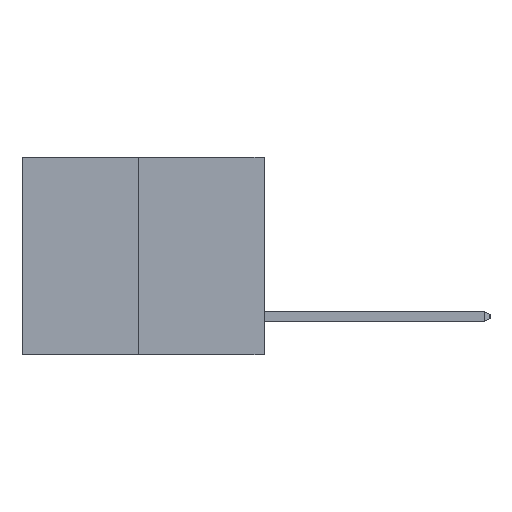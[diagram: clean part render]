
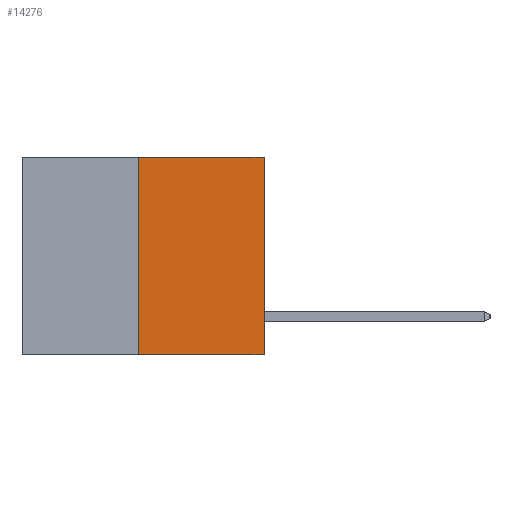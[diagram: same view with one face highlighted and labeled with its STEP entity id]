
A CAD part, left-side view. The second image highlights one B-rep face of the part: STEP entity #14276.
In plain terms, the highlighted planar face has unit normal (-1, 0, 0).
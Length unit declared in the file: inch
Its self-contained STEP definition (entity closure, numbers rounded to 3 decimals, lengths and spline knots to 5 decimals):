
#96 = ORIENTED_EDGE ( 'NONE', *, *, #14423, .F. ) ;
#719 = LINE ( 'NONE', #15150, #18676 ) ;
#1601 = EDGE_CURVE ( 'NONE', #19548, #9227, #719, .T. ) ;
#2883 = LINE ( 'NONE', #22093, #15667 ) ;
#3592 = DIRECTION ( 'NONE',  ( 0., -1., 0. ) ) ;
#3836 = AXIS2_PLACEMENT_3D ( 'NONE', #12516, #15598, #21388 ) ;
#4018 = CARTESIAN_POINT ( 'NONE',  ( 0., 0.312, 0. ) ) ;
#4059 = EDGE_LOOP ( 'NONE', ( #96, #14963, #13814, #21442 ) ) ;
#5556 = PLANE ( 'NONE',  #3836 ) ;
#5925 = VECTOR ( 'NONE', #3592, 39.37008 ) ;
#6572 = EDGE_CURVE ( 'NONE', #9227, #20650, #2883, .T. ) ;
#7530 = FACE_OUTER_BOUND ( 'NONE', #4059, .T. ) ;
#8862 = DIRECTION ( 'NONE',  ( 0., 0., 1. ) ) ;
#9227 = VERTEX_POINT ( 'NONE', #14667 ) ;
#9747 = DIRECTION ( 'NONE',  ( 0., 0., 1. ) ) ;
#10704 = VERTEX_POINT ( 'NONE', #4018 ) ;
#11401 = DIRECTION ( 'NONE',  ( 0., -1., 0. ) ) ;
#12516 = CARTESIAN_POINT ( 'NONE',  ( 0., 0.6, 0. ) ) ;
#13814 = ORIENTED_EDGE ( 'NONE', *, *, #6572, .T. ) ;
#13989 = CARTESIAN_POINT ( 'NONE',  ( 0., 0.6, 0. ) ) ;
#14276 = ADVANCED_FACE ( 'NONE', ( #7530 ), #5556, .F. ) ;
#14423 = EDGE_CURVE ( 'NONE', #19548, #10704, #15429, .T. ) ;
#14667 = CARTESIAN_POINT ( 'NONE',  ( 0., 0., -0.49 ) ) ;
#14963 = ORIENTED_EDGE ( 'NONE', *, *, #1601, .T. ) ;
#15150 = CARTESIAN_POINT ( 'NONE',  ( 0., 0.6, -0.49 ) ) ;
#15429 = LINE ( 'NONE', #19310, #17905 ) ;
#15598 = DIRECTION ( 'NONE',  ( 1., 0., 0. ) ) ;
#15667 = VECTOR ( 'NONE', #9747, 39.37008 ) ;
#15998 = LINE ( 'NONE', #13989, #5925 ) ;
#16375 = EDGE_CURVE ( 'NONE', #10704, #20650, #15998, .T. ) ;
#16965 = CARTESIAN_POINT ( 'NONE',  ( 0., 0., 0. ) ) ;
#17905 = VECTOR ( 'NONE', #8862, 39.37008 ) ;
#18676 = VECTOR ( 'NONE', #11401, 39.37008 ) ;
#19310 = CARTESIAN_POINT ( 'NONE',  ( 0., 0.312, -0.49 ) ) ;
#19548 = VERTEX_POINT ( 'NONE', #20708 ) ;
#20650 = VERTEX_POINT ( 'NONE', #16965 ) ;
#20708 = CARTESIAN_POINT ( 'NONE',  ( 0., 0.312, -0.49 ) ) ;
#21388 = DIRECTION ( 'NONE',  ( 0., 0., -1. ) ) ;
#21442 = ORIENTED_EDGE ( 'NONE', *, *, #16375, .F. ) ;
#22093 = CARTESIAN_POINT ( 'NONE',  ( 0., 0., 0. ) ) ;
